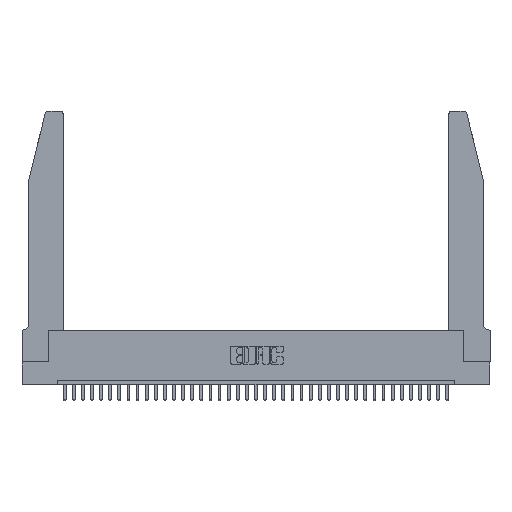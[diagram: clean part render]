
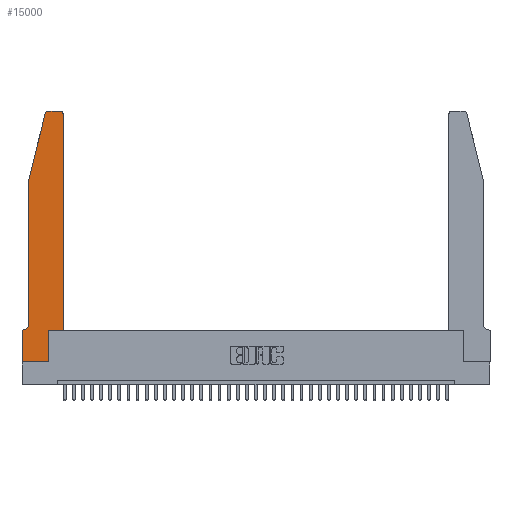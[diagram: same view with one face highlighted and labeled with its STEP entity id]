
A CAD part, top view. The second image highlights one B-rep face of the part: STEP entity #15000.
In plain terms, the highlighted planar face has unit normal (0, 0, 1).
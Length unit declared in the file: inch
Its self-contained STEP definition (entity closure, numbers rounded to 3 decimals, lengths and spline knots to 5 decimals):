
#577 = CIRCLE ( 'NONE', #31671, 0.03 ) ;
#695 = EDGE_CURVE ( 'NONE', #14454, #13355, #18622, .T. ) ;
#746 = VERTEX_POINT ( 'NONE', #31227 ) ;
#982 = CIRCLE ( 'NONE', #9465, 0.03 ) ;
#1259 = VECTOR ( 'NONE', #24552, 39.37008 ) ;
#1409 = DIRECTION ( 'NONE',  ( 1., 0., 0. ) ) ;
#1544 = DIRECTION ( 'NONE',  ( 0., 1., 0. ) ) ;
#2451 = LINE ( 'NONE', #15719, #14093 ) ;
#2660 = CARTESIAN_POINT ( 'NONE',  ( 0.0055, 0.42, 0.37 ) ) ;
#2667 = VECTOR ( 'NONE', #34106, 39.37008 ) ;
#3078 = VERTEX_POINT ( 'NONE', #32509 ) ;
#3189 = ORIENTED_EDGE ( 'NONE', *, *, #23804, .T. ) ;
#3629 = DIRECTION ( 'NONE',  ( -1., 0., 0. ) ) ;
#3866 = ORIENTED_EDGE ( 'NONE', *, *, #6229, .T. ) ;
#4340 = VECTOR ( 'NONE', #1544, 39.37008 ) ;
#5277 = DIRECTION ( 'NONE',  ( 0., 0., 1. ) ) ;
#5422 = ORIENTED_EDGE ( 'NONE', *, *, #6337, .T. ) ;
#5925 = DIRECTION ( 'NONE',  ( -0.239, -0.971, 0. ) ) ;
#6229 = EDGE_CURVE ( 'NONE', #3078, #28619, #23205, .T. ) ;
#6337 = EDGE_CURVE ( 'NONE', #20287, #26925, #13798, .T. ) ;
#6349 = FACE_OUTER_BOUND ( 'NONE', #33937, .T. ) ;
#6541 = CARTESIAN_POINT ( 'NONE',  ( 0.4505, 2.72, 0.37 ) ) ;
#6644 = CARTESIAN_POINT ( 'NONE',  ( 0.4505, 0.35, 0.37 ) ) ;
#8198 = ORIENTED_EDGE ( 'NONE', *, *, #695, .T. ) ;
#8607 = VECTOR ( 'NONE', #3629, 39.37008 ) ;
#9321 = EDGE_CURVE ( 'NONE', #28619, #746, #577, .T. ) ;
#9465 = AXIS2_PLACEMENT_3D ( 'NONE', #22556, #25364, #28267 ) ;
#9516 = VERTEX_POINT ( 'NONE', #29191 ) ;
#10196 = VECTOR ( 'NONE', #5925, 39.37008 ) ;
#10447 = EDGE_CURVE ( 'NONE', #13355, #9516, #22063, .T. ) ;
#10779 = VERTEX_POINT ( 'NONE', #20594 ) ;
#11666 = LINE ( 'NONE', #6644, #19293 ) ;
#12088 = DIRECTION ( 'NONE',  ( -1., 0., 0. ) ) ;
#12557 = EDGE_CURVE ( 'NONE', #23960, #35931, #21377, .T. ) ;
#13125 = DIRECTION ( 'NONE',  ( 0., -1., 0. ) ) ;
#13355 = VERTEX_POINT ( 'NONE', #36314 ) ;
#13552 = VECTOR ( 'NONE', #13125, 39.37008 ) ;
#13569 = DIRECTION ( 'NONE',  ( 1., 0., 0. ) ) ;
#13798 = LINE ( 'NONE', #36761, #10196 ) ;
#13915 = CARTESIAN_POINT ( 'NONE',  ( 0., 0., 0.37 ) ) ;
#14093 = VECTOR ( 'NONE', #18342, 39.37008 ) ;
#14142 = ORIENTED_EDGE ( 'NONE', *, *, #36510, .T. ) ;
#14175 = DIRECTION ( 'NONE',  ( 0., 0., -1. ) ) ;
#14228 = AXIS2_PLACEMENT_3D ( 'NONE', #2660, #14175, #28325 ) ;
#14454 = VERTEX_POINT ( 'NONE', #30835 ) ;
#14885 = CARTESIAN_POINT ( 'NONE',  ( 0.0755, 2., 0.37 ) ) ;
#14989 = CARTESIAN_POINT ( 'NONE',  ( 0.2865, 0., 0.37 ) ) ;
#15000 = ADVANCED_FACE ( 'NONE', ( #6349 ), #29279, .T. ) ;
#15314 = LINE ( 'NONE', #30802, #13552 ) ;
#15370 = ORIENTED_EDGE ( 'NONE', *, *, #20745, .T. ) ;
#15719 = CARTESIAN_POINT ( 'NONE',  ( 0., 0., 0.37 ) ) ;
#15938 = CARTESIAN_POINT ( 'NONE',  ( 0., 0., 0.37 ) ) ;
#18342 = DIRECTION ( 'NONE',  ( 0., -1., 0. ) ) ;
#18622 = CIRCLE ( 'NONE', #14228, 0.07 ) ;
#19293 = VECTOR ( 'NONE', #1409, 39.37008 ) ;
#19332 = AXIS2_PLACEMENT_3D ( 'NONE', #34941, #35067, #26259 ) ;
#20287 = VERTEX_POINT ( 'NONE', #25016 ) ;
#20594 = CARTESIAN_POINT ( 'NONE',  ( 0.284, 2.75, 0.37 ) ) ;
#20745 = EDGE_CURVE ( 'NONE', #9516, #35659, #2451, .T. ) ;
#20794 = CARTESIAN_POINT ( 'NONE',  ( 0.0755, 0.35, 0.37 ) ) ;
#21231 = ORIENTED_EDGE ( 'NONE', *, *, #9321, .T. ) ;
#21377 = LINE ( 'NONE', #35745, #4340 ) ;
#21621 = CARTESIAN_POINT ( 'NONE',  ( 0.4505, 0.35, 0.37 ) ) ;
#22063 = LINE ( 'NONE', #20794, #8607 ) ;
#22556 = CARTESIAN_POINT ( 'NONE',  ( 0.284, 2.72, 0.37 ) ) ;
#23205 = LINE ( 'NONE', #21621, #1259 ) ;
#23804 = EDGE_CURVE ( 'NONE', #35659, #23960, #30459, .T. ) ;
#23960 = VERTEX_POINT ( 'NONE', #14989 ) ;
#24410 = EDGE_CURVE ( 'NONE', #10779, #20287, #982, .T. ) ;
#24459 = ORIENTED_EDGE ( 'NONE', *, *, #10447, .T. ) ;
#24552 = DIRECTION ( 'NONE',  ( 0., 1., 0. ) ) ;
#25016 = CARTESIAN_POINT ( 'NONE',  ( 0.25487, 2.72718, 0.37 ) ) ;
#25364 = DIRECTION ( 'NONE',  ( 0., 0., 1. ) ) ;
#26259 = DIRECTION ( 'NONE',  ( 1., 0., 0. ) ) ;
#26639 = ORIENTED_EDGE ( 'NONE', *, *, #12557, .T. ) ;
#26925 = VERTEX_POINT ( 'NONE', #14885 ) ;
#27361 = CARTESIAN_POINT ( 'NONE',  ( 0.2865, 0.35, 0.37 ) ) ;
#28267 = DIRECTION ( 'NONE',  ( 1., 0., 0. ) ) ;
#28325 = DIRECTION ( 'NONE',  ( -1., 0., 0. ) ) ;
#28619 = VERTEX_POINT ( 'NONE', #6541 ) ;
#29191 = CARTESIAN_POINT ( 'NONE',  ( 0., 0.35, 0.37 ) ) ;
#29279 = PLANE ( 'NONE',  #19332 ) ;
#30424 = EDGE_CURVE ( 'NONE', #746, #10779, #36756, .T. ) ;
#30459 = LINE ( 'NONE', #15938, #2667 ) ;
#30738 = CARTESIAN_POINT ( 'NONE',  ( 0.4205, 2.72, 0.37 ) ) ;
#30802 = CARTESIAN_POINT ( 'NONE',  ( 0.0755, 2., 0.37 ) ) ;
#30835 = CARTESIAN_POINT ( 'NONE',  ( 0.0755, 0.42, 0.37 ) ) ;
#31196 = EDGE_CURVE ( 'NONE', #35931, #3078, #11666, .T. ) ;
#31227 = CARTESIAN_POINT ( 'NONE',  ( 0.4205, 2.75, 0.37 ) ) ;
#31671 = AXIS2_PLACEMENT_3D ( 'NONE', #30738, #5277, #13569 ) ;
#32300 = ORIENTED_EDGE ( 'NONE', *, *, #30424, .T. ) ;
#32509 = CARTESIAN_POINT ( 'NONE',  ( 0.4505, 0.35, 0.37 ) ) ;
#33518 = ORIENTED_EDGE ( 'NONE', *, *, #31196, .T. ) ;
#33937 = EDGE_LOOP ( 'NONE', ( #32300, #34690, #5422, #14142, #8198, #24459, #15370, #3189, #26639, #33518, #3866, #21231 ) ) ;
#34083 = VECTOR ( 'NONE', #12088, 39.37008 ) ;
#34106 = DIRECTION ( 'NONE',  ( 1., 0., 0. ) ) ;
#34690 = ORIENTED_EDGE ( 'NONE', *, *, #24410, .T. ) ;
#34893 = CARTESIAN_POINT ( 'NONE',  ( 0.2605, 2.75, 0.37 ) ) ;
#34941 = CARTESIAN_POINT ( 'NONE',  ( 0., 0.35, 0.37 ) ) ;
#35067 = DIRECTION ( 'NONE',  ( 0., 0., 1. ) ) ;
#35659 = VERTEX_POINT ( 'NONE', #13915 ) ;
#35745 = CARTESIAN_POINT ( 'NONE',  ( 0.2865, 0.35, 0.37 ) ) ;
#35931 = VERTEX_POINT ( 'NONE', #27361 ) ;
#36314 = CARTESIAN_POINT ( 'NONE',  ( 0.0055, 0.35, 0.37 ) ) ;
#36510 = EDGE_CURVE ( 'NONE', #26925, #14454, #15314, .T. ) ;
#36756 = LINE ( 'NONE', #34893, #34083 ) ;
#36761 = CARTESIAN_POINT ( 'NONE',  ( 0.0755, 2., 0.37 ) ) ;
